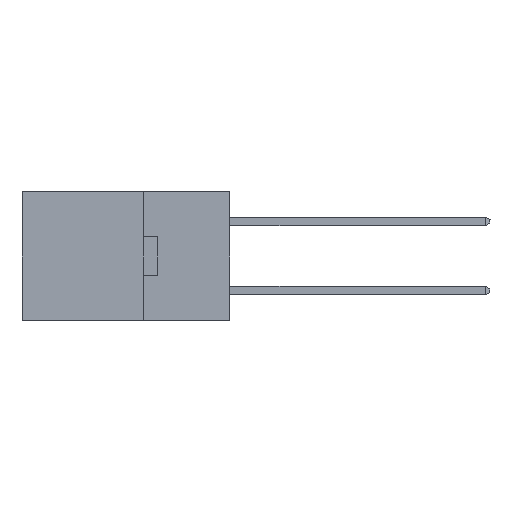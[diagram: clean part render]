
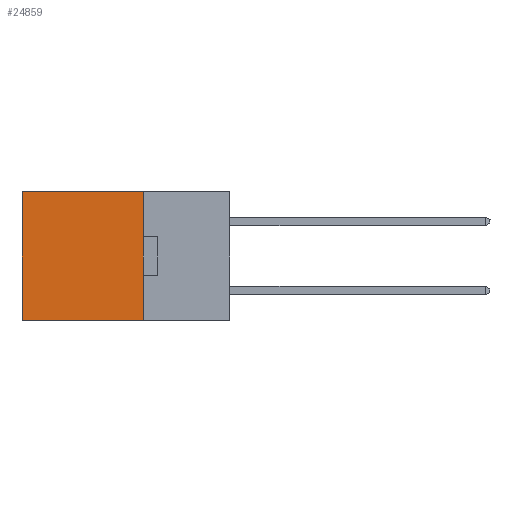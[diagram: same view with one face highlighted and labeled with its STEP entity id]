
A CAD part, left-side view. The second image highlights one B-rep face of the part: STEP entity #24859.
In plain terms, the highlighted planar face has unit normal (-1, 0, 0).
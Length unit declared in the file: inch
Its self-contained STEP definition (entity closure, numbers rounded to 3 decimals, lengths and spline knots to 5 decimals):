
#994 = DIRECTION ( 'NONE',  ( 0., 0., -1. ) ) ;
#3552 = CARTESIAN_POINT ( 'NONE',  ( 0.2615, 0.6, -0.37 ) ) ;
#3900 = ORIENTED_EDGE ( 'NONE', *, *, #10684, .T. ) ;
#5079 = LINE ( 'NONE', #27201, #9860 ) ;
#5631 = DIRECTION ( 'NONE',  ( 0., 0., -1. ) ) ;
#6247 = CARTESIAN_POINT ( 'NONE',  ( 0.2615, 0.25, 0. ) ) ;
#6537 = DIRECTION ( 'NONE',  ( 0., 1., 0. ) ) ;
#8587 = AXIS2_PLACEMENT_3D ( 'NONE', #12004, #16602, #994 ) ;
#8650 = VERTEX_POINT ( 'NONE', #3552 ) ;
#9206 = DIRECTION ( 'NONE',  ( 0., 1., 0. ) ) ;
#9860 = VECTOR ( 'NONE', #5631, 39.37008 ) ;
#9957 = VECTOR ( 'NONE', #19649, 39.37008 ) ;
#10190 = EDGE_CURVE ( 'NONE', #11187, #17726, #23537, .T. ) ;
#10378 = CARTESIAN_POINT ( 'NONE',  ( 0.2615, 0.25, -0.37 ) ) ;
#10684 = EDGE_CURVE ( 'NONE', #11187, #26427, #26034, .T. ) ;
#11073 = CARTESIAN_POINT ( 'NONE',  ( 0.2615, 0.25, -0.37 ) ) ;
#11187 = VERTEX_POINT ( 'NONE', #14313 ) ;
#11214 = LINE ( 'NONE', #11073, #20824 ) ;
#12004 = CARTESIAN_POINT ( 'NONE',  ( 0.2615, 0.25, -0.37 ) ) ;
#12841 = ORIENTED_EDGE ( 'NONE', *, *, #15382, .F. ) ;
#14313 = CARTESIAN_POINT ( 'NONE',  ( 0.2615, 0.25, 0. ) ) ;
#14318 = CARTESIAN_POINT ( 'NONE',  ( 0.2615, 0.25, -0.37 ) ) ;
#14447 = ORIENTED_EDGE ( 'NONE', *, *, #10190, .F. ) ;
#15382 = EDGE_CURVE ( 'NONE', #17726, #8650, #11214, .T. ) ;
#16602 = DIRECTION ( 'NONE',  ( 1., 0., 0. ) ) ;
#17726 = VERTEX_POINT ( 'NONE', #14318 ) ;
#18069 = CARTESIAN_POINT ( 'NONE',  ( 0.2615, 0.6, 0. ) ) ;
#19190 = EDGE_CURVE ( 'NONE', #26427, #8650, #5079, .T. ) ;
#19649 = DIRECTION ( 'NONE',  ( 0., 0., -1. ) ) ;
#20824 = VECTOR ( 'NONE', #9206, 39.37008 ) ;
#22986 = FACE_OUTER_BOUND ( 'NONE', #24575, .T. ) ;
#23537 = LINE ( 'NONE', #10378, #9957 ) ;
#24308 = VECTOR ( 'NONE', #6537, 39.37008 ) ;
#24575 = EDGE_LOOP ( 'NONE', ( #25376, #12841, #14447, #3900 ) ) ;
#24859 = ADVANCED_FACE ( 'NONE', ( #22986 ), #25423, .F. ) ;
#25376 = ORIENTED_EDGE ( 'NONE', *, *, #19190, .T. ) ;
#25423 = PLANE ( 'NONE',  #8587 ) ;
#26034 = LINE ( 'NONE', #6247, #24308 ) ;
#26427 = VERTEX_POINT ( 'NONE', #18069 ) ;
#27201 = CARTESIAN_POINT ( 'NONE',  ( 0.2615, 0.6, -0.37 ) ) ;
